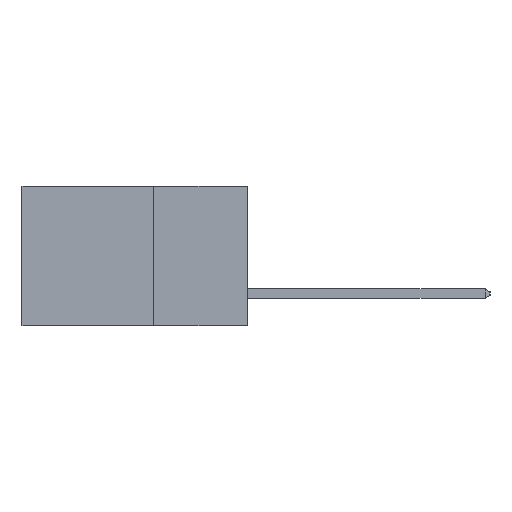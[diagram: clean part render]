
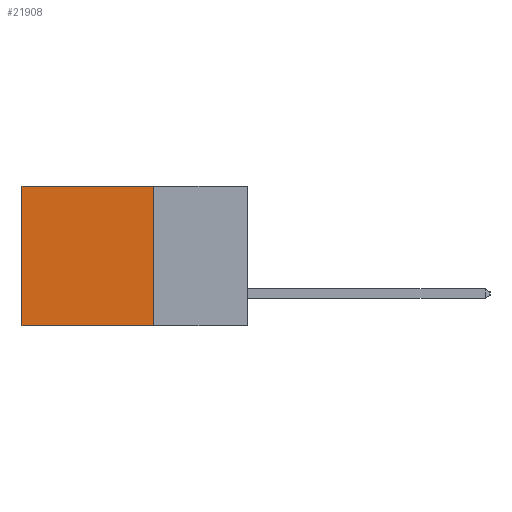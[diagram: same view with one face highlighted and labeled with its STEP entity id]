
A CAD part, left-side view. The second image highlights one B-rep face of the part: STEP entity #21908.
In plain terms, the highlighted planar face has unit normal (-1, 0, 0).
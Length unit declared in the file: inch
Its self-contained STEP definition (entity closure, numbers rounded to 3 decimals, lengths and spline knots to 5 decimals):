
#787 = CARTESIAN_POINT ( 'NONE',  ( 0.298, 0.6, 0. ) ) ;
#1155 = CARTESIAN_POINT ( 'NONE',  ( 0.298, 0.25, 0. ) ) ;
#1157 = VECTOR ( 'NONE', #11026, 39.37008 ) ;
#2551 = LINE ( 'NONE', #18006, #22550 ) ;
#2749 = CARTESIAN_POINT ( 'NONE',  ( 0.298, 0.25, 0. ) ) ;
#2818 = CARTESIAN_POINT ( 'NONE',  ( 0.298, 0.25, -0.37 ) ) ;
#5944 = VERTEX_POINT ( 'NONE', #787 ) ;
#6476 = LINE ( 'NONE', #1155, #1157 ) ;
#6972 = FACE_OUTER_BOUND ( 'NONE', #18522, .T. ) ;
#7067 = CARTESIAN_POINT ( 'NONE',  ( 0.298, 0.6, -0.37 ) ) ;
#8172 = CARTESIAN_POINT ( 'NONE',  ( 0.298, 0.25, -0.37 ) ) ;
#8722 = PLANE ( 'NONE',  #15906 ) ;
#10028 = LINE ( 'NONE', #21827, #19635 ) ;
#10396 = DIRECTION ( 'NONE',  ( 0., 0., -1. ) ) ;
#10410 = ORIENTED_EDGE ( 'NONE', *, *, #22503, .T. ) ;
#10675 = DIRECTION ( 'NONE',  ( 0., 0., -1. ) ) ;
#11026 = DIRECTION ( 'NONE',  ( 0., 0., -1. ) ) ;
#11788 = ORIENTED_EDGE ( 'NONE', *, *, #16125, .T. ) ;
#11859 = VERTEX_POINT ( 'NONE', #15010 ) ;
#14540 = ORIENTED_EDGE ( 'NONE', *, *, #15156, .F. ) ;
#15010 = CARTESIAN_POINT ( 'NONE',  ( 0.298, 0.25, 0. ) ) ;
#15156 = EDGE_CURVE ( 'NONE', #11859, #21818, #6476, .T. ) ;
#15906 = AXIS2_PLACEMENT_3D ( 'NONE', #2749, #22170, #10675 ) ;
#16085 = DIRECTION ( 'NONE',  ( 0., 1., 0. ) ) ;
#16125 = EDGE_CURVE ( 'NONE', #11859, #5944, #10028, .T. ) ;
#18006 = CARTESIAN_POINT ( 'NONE',  ( 0.298, 0.6, 0. ) ) ;
#18522 = EDGE_LOOP ( 'NONE', ( #10410, #19479, #14540, #11788 ) ) ;
#18840 = VECTOR ( 'NONE', #22227, 39.37008 ) ;
#19479 = ORIENTED_EDGE ( 'NONE', *, *, #24907, .F. ) ;
#19635 = VECTOR ( 'NONE', #16085, 39.37008 ) ;
#21818 = VERTEX_POINT ( 'NONE', #8172 ) ;
#21827 = CARTESIAN_POINT ( 'NONE',  ( 0.298, 0.25, 0. ) ) ;
#21908 = ADVANCED_FACE ( 'NONE', ( #6972 ), #8722, .F. ) ;
#22170 = DIRECTION ( 'NONE',  ( 1., 0., 0. ) ) ;
#22227 = DIRECTION ( 'NONE',  ( 0., 1., 0. ) ) ;
#22503 = EDGE_CURVE ( 'NONE', #5944, #23237, #2551, .T. ) ;
#22550 = VECTOR ( 'NONE', #10396, 39.37008 ) ;
#22807 = LINE ( 'NONE', #2818, #18840 ) ;
#23237 = VERTEX_POINT ( 'NONE', #7067 ) ;
#24907 = EDGE_CURVE ( 'NONE', #21818, #23237, #22807, .T. ) ;
